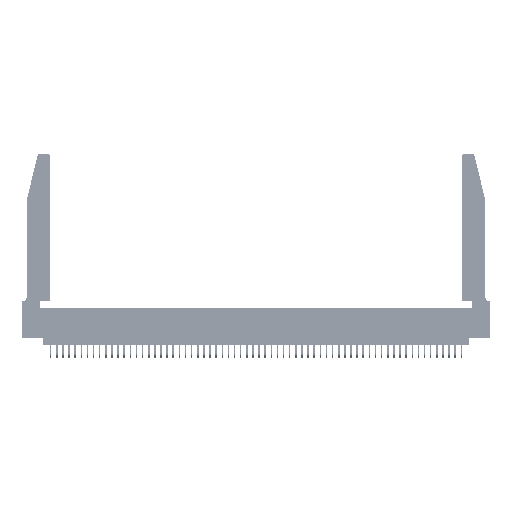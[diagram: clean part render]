
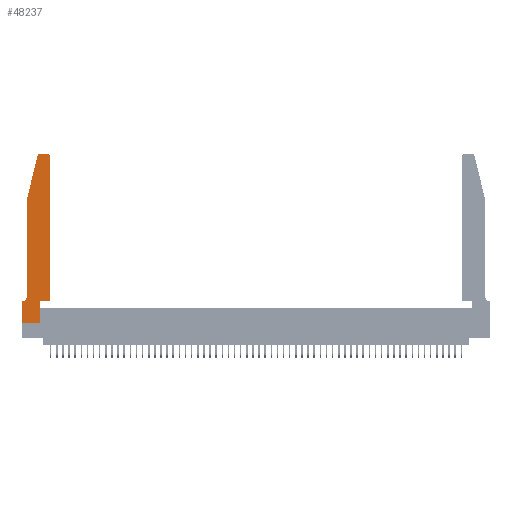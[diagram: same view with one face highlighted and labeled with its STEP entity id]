
A CAD part, top view. The second image highlights one B-rep face of the part: STEP entity #48237.
In plain terms, the highlighted planar face has unit normal (0, 0, 1).
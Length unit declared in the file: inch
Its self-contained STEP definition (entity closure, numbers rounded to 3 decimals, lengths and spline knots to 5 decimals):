
#68 = CARTESIAN_POINT ( 'NONE',  ( 0.0055, 0.35, 0.37 ) ) ;
#2168 = LINE ( 'NONE', #20738, #21264 ) ;
#2640 = LINE ( 'NONE', #52963, #25115 ) ;
#3070 = ORIENTED_EDGE ( 'NONE', *, *, #55697, .T. ) ;
#3219 = LINE ( 'NONE', #44084, #23682 ) ;
#3721 = AXIS2_PLACEMENT_3D ( 'NONE', #24784, #20418, #55254 ) ;
#4392 = VECTOR ( 'NONE', #46472, 39.37008 ) ;
#4401 = DIRECTION ( 'NONE',  ( 1., 0., 0. ) ) ;
#4838 = DIRECTION ( 'NONE',  ( -1., 0., 0. ) ) ;
#5484 = PLANE ( 'NONE',  #49071 ) ;
#5722 = EDGE_CURVE ( 'NONE', #55264, #27678, #27182, .T. ) ;
#8877 = EDGE_CURVE ( 'NONE', #14649, #18382, #16480, .T. ) ;
#9797 = EDGE_CURVE ( 'NONE', #36008, #32037, #14318, .T. ) ;
#10205 = CARTESIAN_POINT ( 'NONE',  ( 0., 0., 0.37 ) ) ;
#10212 = LINE ( 'NONE', #29319, #4392 ) ;
#10919 = ORIENTED_EDGE ( 'NONE', *, *, #30097, .T. ) ;
#12208 = CARTESIAN_POINT ( 'NONE',  ( 0.2865, 0.35, 0.37 ) ) ;
#12619 = LINE ( 'NONE', #53316, #48121 ) ;
#12752 = CARTESIAN_POINT ( 'NONE',  ( 0.0055, 0.42, 0.37 ) ) ;
#13224 = VECTOR ( 'NONE', #34120, 39.37008 ) ;
#13472 = AXIS2_PLACEMENT_3D ( 'NONE', #25573, #52068, #4401 ) ;
#14318 = CIRCLE ( 'NONE', #3721, 0.03 ) ;
#14649 = VERTEX_POINT ( 'NONE', #12208 ) ;
#14939 = DIRECTION ( 'NONE',  ( 0., 1., 0. ) ) ;
#15318 = VERTEX_POINT ( 'NONE', #45992 ) ;
#15745 = ORIENTED_EDGE ( 'NONE', *, *, #52436, .T. ) ;
#15804 = VERTEX_POINT ( 'NONE', #35463 ) ;
#16480 = LINE ( 'NONE', #18963, #35527 ) ;
#16887 = VERTEX_POINT ( 'NONE', #52516 ) ;
#17277 = ORIENTED_EDGE ( 'NONE', *, *, #48887, .T. ) ;
#18382 = VERTEX_POINT ( 'NONE', #45529 ) ;
#18631 = LINE ( 'NONE', #41018, #37051 ) ;
#18963 = CARTESIAN_POINT ( 'NONE',  ( 0.4505, 0.35, 0.37 ) ) ;
#19960 = ORIENTED_EDGE ( 'NONE', *, *, #9797, .T. ) ;
#20418 = DIRECTION ( 'NONE',  ( 0., 0., 1. ) ) ;
#20489 = ORIENTED_EDGE ( 'NONE', *, *, #8877, .T. ) ;
#20738 = CARTESIAN_POINT ( 'NONE',  ( 0.2865, 0.35, 0.37 ) ) ;
#21264 = VECTOR ( 'NONE', #46448, 39.37008 ) ;
#23327 = EDGE_LOOP ( 'NONE', ( #45951, #40542, #3070, #47857, #25793, #15745, #17277, #40277, #10919, #20489, #45158, #19960 ) ) ;
#23542 = LINE ( 'NONE', #10205, #38572 ) ;
#23682 = VECTOR ( 'NONE', #4838, 39.37008 ) ;
#24784 = CARTESIAN_POINT ( 'NONE',  ( 0.4205, 2.72, 0.37 ) ) ;
#25115 = VECTOR ( 'NONE', #31029, 39.37008 ) ;
#25142 = CARTESIAN_POINT ( 'NONE',  ( 0., 0.35, 0.37 ) ) ;
#25573 = CARTESIAN_POINT ( 'NONE',  ( 0.284, 2.72, 0.37 ) ) ;
#25793 = ORIENTED_EDGE ( 'NONE', *, *, #55578, .T. ) ;
#25828 = EDGE_CURVE ( 'NONE', #15318, #15804, #10212, .T. ) ;
#27182 = CIRCLE ( 'NONE', #13472, 0.03 ) ;
#27346 = DIRECTION ( 'NONE',  ( 1., 0., 0. ) ) ;
#27418 = DIRECTION ( 'NONE',  ( 1., 0., 0. ) ) ;
#27678 = VERTEX_POINT ( 'NONE', #31160 ) ;
#28192 = VERTEX_POINT ( 'NONE', #68 ) ;
#29319 = CARTESIAN_POINT ( 'NONE',  ( 0., 0., 0.37 ) ) ;
#30097 = EDGE_CURVE ( 'NONE', #15804, #14649, #2168, .T. ) ;
#31029 = DIRECTION ( 'NONE',  ( -0.239, -0.971, 0. ) ) ;
#31160 = CARTESIAN_POINT ( 'NONE',  ( 0.25487, 2.72718, 0.37 ) ) ;
#31698 = FACE_OUTER_BOUND ( 'NONE', #23327, .T. ) ;
#32037 = VERTEX_POINT ( 'NONE', #52914 ) ;
#34120 = DIRECTION ( 'NONE',  ( 0., -1., 0. ) ) ;
#35463 = CARTESIAN_POINT ( 'NONE',  ( 0.2865, 0., 0.37 ) ) ;
#35527 = VECTOR ( 'NONE', #27346, 39.37008 ) ;
#36008 = VERTEX_POINT ( 'NONE', #44371 ) ;
#37051 = VECTOR ( 'NONE', #14939, 39.37008 ) ;
#37065 = EDGE_CURVE ( 'NONE', #42422, #16887, #52131, .T. ) ;
#38158 = CARTESIAN_POINT ( 'NONE',  ( 0.0755, 2., 0.37 ) ) ;
#38572 = VECTOR ( 'NONE', #40670, 39.37008 ) ;
#40277 = ORIENTED_EDGE ( 'NONE', *, *, #25828, .T. ) ;
#40542 = ORIENTED_EDGE ( 'NONE', *, *, #5722, .T. ) ;
#40670 = DIRECTION ( 'NONE',  ( 0., -1., 0. ) ) ;
#41018 = CARTESIAN_POINT ( 'NONE',  ( 0.4505, 0.35, 0.37 ) ) ;
#41934 = AXIS2_PLACEMENT_3D ( 'NONE', #12752, #56197, #52222 ) ;
#42422 = VERTEX_POINT ( 'NONE', #45545 ) ;
#42560 = VERTEX_POINT ( 'NONE', #25142 ) ;
#43509 = CIRCLE ( 'NONE', #41934, 0.07 ) ;
#43694 = EDGE_CURVE ( 'NONE', #18382, #36008, #18631, .T. ) ;
#44084 = CARTESIAN_POINT ( 'NONE',  ( 0.2605, 2.75, 0.37 ) ) ;
#44345 = CARTESIAN_POINT ( 'NONE',  ( 0., 0.35, 0.37 ) ) ;
#44371 = CARTESIAN_POINT ( 'NONE',  ( 0.4505, 2.72, 0.37 ) ) ;
#44726 = DIRECTION ( 'NONE',  ( 0., 0., 1. ) ) ;
#45158 = ORIENTED_EDGE ( 'NONE', *, *, #43694, .T. ) ;
#45529 = CARTESIAN_POINT ( 'NONE',  ( 0.4505, 0.35, 0.37 ) ) ;
#45545 = CARTESIAN_POINT ( 'NONE',  ( 0.0755, 2., 0.37 ) ) ;
#45951 = ORIENTED_EDGE ( 'NONE', *, *, #46788, .T. ) ;
#45992 = CARTESIAN_POINT ( 'NONE',  ( 0., 0., 0.37 ) ) ;
#46448 = DIRECTION ( 'NONE',  ( 0., 1., 0. ) ) ;
#46472 = DIRECTION ( 'NONE',  ( 1., 0., 0. ) ) ;
#46788 = EDGE_CURVE ( 'NONE', #32037, #55264, #3219, .T. ) ;
#47857 = ORIENTED_EDGE ( 'NONE', *, *, #37065, .T. ) ;
#48121 = VECTOR ( 'NONE', #49289, 39.37008 ) ;
#48237 = ADVANCED_FACE ( 'NONE', ( #31698 ), #5484, .T. ) ;
#48887 = EDGE_CURVE ( 'NONE', #42560, #15318, #23542, .T. ) ;
#49071 = AXIS2_PLACEMENT_3D ( 'NONE', #44345, #44726, #27418 ) ;
#49289 = DIRECTION ( 'NONE',  ( -1., 0., 0. ) ) ;
#52068 = DIRECTION ( 'NONE',  ( 0., 0., 1. ) ) ;
#52131 = LINE ( 'NONE', #38158, #13224 ) ;
#52222 = DIRECTION ( 'NONE',  ( -1., 0., 0. ) ) ;
#52436 = EDGE_CURVE ( 'NONE', #28192, #42560, #12619, .T. ) ;
#52516 = CARTESIAN_POINT ( 'NONE',  ( 0.0755, 0.42, 0.37 ) ) ;
#52914 = CARTESIAN_POINT ( 'NONE',  ( 0.4205, 2.75, 0.37 ) ) ;
#52963 = CARTESIAN_POINT ( 'NONE',  ( 0.0755, 2., 0.37 ) ) ;
#53316 = CARTESIAN_POINT ( 'NONE',  ( 0.0755, 0.35, 0.37 ) ) ;
#54520 = CARTESIAN_POINT ( 'NONE',  ( 0.284, 2.75, 0.37 ) ) ;
#55254 = DIRECTION ( 'NONE',  ( 1., 0., 0. ) ) ;
#55264 = VERTEX_POINT ( 'NONE', #54520 ) ;
#55578 = EDGE_CURVE ( 'NONE', #16887, #28192, #43509, .T. ) ;
#55697 = EDGE_CURVE ( 'NONE', #27678, #42422, #2640, .T. ) ;
#56197 = DIRECTION ( 'NONE',  ( 0., 0., -1. ) ) ;
